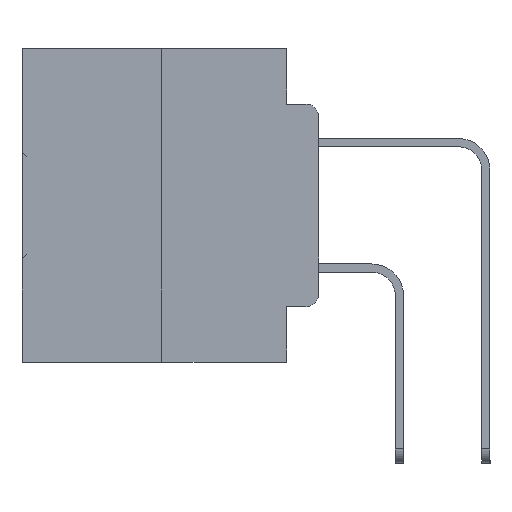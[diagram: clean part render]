
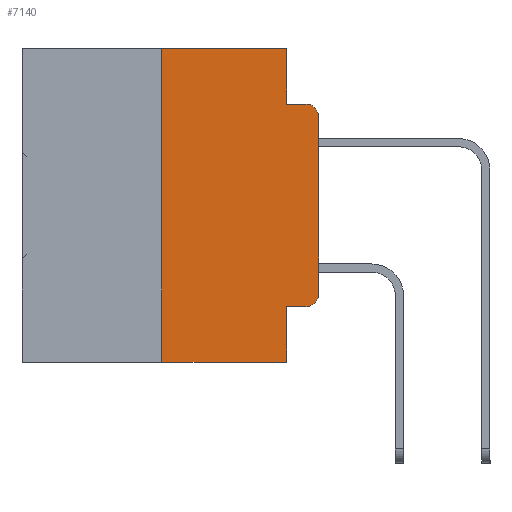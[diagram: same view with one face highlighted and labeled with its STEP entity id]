
A CAD part, left-side view. The second image highlights one B-rep face of the part: STEP entity #7140.
In plain terms, the highlighted planar face has unit normal (-1, 0, 0).
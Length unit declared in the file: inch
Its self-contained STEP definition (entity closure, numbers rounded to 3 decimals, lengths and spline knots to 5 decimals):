
#17 = LINE ( 'NONE', #10587, #12232 ) ;
#778 = VECTOR ( 'NONE', #29544, 39.37008 ) ;
#1004 = VERTEX_POINT ( 'NONE', #22967 ) ;
#1310 = VECTOR ( 'NONE', #13694, 39.37008 ) ;
#1655 = LINE ( 'NONE', #13505, #778 ) ;
#2083 = CIRCLE ( 'NONE', #3443, 0.02 ) ;
#2394 = LINE ( 'NONE', #18961, #31163 ) ;
#2472 = DIRECTION ( 'NONE',  ( 0., -1., 0. ) ) ;
#3310 = CARTESIAN_POINT ( 'NONE',  ( 0., 0.051, 0. ) ) ;
#3443 = AXIS2_PLACEMENT_3D ( 'NONE', #24940, #8804, #27569 ) ;
#3861 = VERTEX_POINT ( 'NONE', #34736 ) ;
#4804 = ORIENTED_EDGE ( 'NONE', *, *, #18585, .T. ) ;
#5105 = DIRECTION ( 'NONE',  ( 0., -1., 0. ) ) ;
#5783 = EDGE_CURVE ( 'NONE', #22459, #1004, #8733, .T. ) ;
#6427 = EDGE_CURVE ( 'NONE', #22459, #11233, #9134, .T. ) ;
#6548 = ORIENTED_EDGE ( 'NONE', *, *, #19818, .F. ) ;
#7105 = LINE ( 'NONE', #26453, #27702 ) ;
#7137 = EDGE_CURVE ( 'NONE', #7697, #31434, #2083, .T. ) ;
#7140 = ADVANCED_FACE ( 'NONE', ( #8635 ), #22324, .F. ) ;
#7409 = CIRCLE ( 'NONE', #26892, 0.02 ) ;
#7697 = VERTEX_POINT ( 'NONE', #21941 ) ;
#7738 = DIRECTION ( 'NONE',  ( 0., 0., -1. ) ) ;
#8262 = VERTEX_POINT ( 'NONE', #34646 ) ;
#8292 = ORIENTED_EDGE ( 'NONE', *, *, #5783, .T. ) ;
#8513 = VERTEX_POINT ( 'NONE', #3310 ) ;
#8619 = DIRECTION ( 'NONE',  ( 0., 0., 1. ) ) ;
#8635 = FACE_OUTER_BOUND ( 'NONE', #21791, .T. ) ;
#8733 = LINE ( 'NONE', #29514, #1310 ) ;
#8804 = DIRECTION ( 'NONE',  ( -1., 0., 0. ) ) ;
#9050 = AXIS2_PLACEMENT_3D ( 'NONE', #14308, #32871, #17050 ) ;
#9134 = LINE ( 'NONE', #19443, #23517 ) ;
#10149 = LINE ( 'NONE', #29936, #30610 ) ;
#10587 = CARTESIAN_POINT ( 'NONE',  ( 0., 0.051, -0.4115 ) ) ;
#11233 = VERTEX_POINT ( 'NONE', #28579 ) ;
#12182 = ORIENTED_EDGE ( 'NONE', *, *, #33385, .T. ) ;
#12232 = VECTOR ( 'NONE', #5105, 39.37008 ) ;
#13505 = CARTESIAN_POINT ( 'NONE',  ( 0., 0., 0. ) ) ;
#13694 = DIRECTION ( 'NONE',  ( 0., -1., 0. ) ) ;
#14308 = CARTESIAN_POINT ( 'NONE',  ( 0., 0.473, 0. ) ) ;
#16082 = CARTESIAN_POINT ( 'NONE',  ( 0., 0.25, -0.5 ) ) ;
#16399 = DIRECTION ( 'NONE',  ( -1., 0., 0. ) ) ;
#17050 = DIRECTION ( 'NONE',  ( 0., 0., -1. ) ) ;
#18585 = EDGE_CURVE ( 'NONE', #31434, #26821, #1655, .T. ) ;
#18961 = CARTESIAN_POINT ( 'NONE',  ( 0., 0.473, 0. ) ) ;
#19443 = CARTESIAN_POINT ( 'NONE',  ( 0., 0.25, 0. ) ) ;
#19786 = ORIENTED_EDGE ( 'NONE', *, *, #7137, .T. ) ;
#19818 = EDGE_CURVE ( 'NONE', #11233, #8513, #2394, .T. ) ;
#21057 = ORIENTED_EDGE ( 'NONE', *, *, #6427, .F. ) ;
#21791 = EDGE_LOOP ( 'NONE', ( #4804, #12182, #26392, #27194, #6548, #21057, #8292, #24343, #25158, #19786 ) ) ;
#21941 = CARTESIAN_POINT ( 'NONE',  ( 0., 0.02, -0.4115 ) ) ;
#22324 = PLANE ( 'NONE',  #9050 ) ;
#22459 = VERTEX_POINT ( 'NONE', #16082 ) ;
#22967 = CARTESIAN_POINT ( 'NONE',  ( 0., 0.051, -0.5 ) ) ;
#23188 = LINE ( 'NONE', #24961, #30134 ) ;
#23517 = VECTOR ( 'NONE', #8619, 39.37008 ) ;
#24343 = ORIENTED_EDGE ( 'NONE', *, *, #32271, .F. ) ;
#24565 = EDGE_CURVE ( 'NONE', #8513, #3861, #7105, .T. ) ;
#24940 = CARTESIAN_POINT ( 'NONE',  ( 0., 0.02, -0.3915 ) ) ;
#24961 = CARTESIAN_POINT ( 'NONE',  ( 0., 0.051, 0. ) ) ;
#25158 = ORIENTED_EDGE ( 'NONE', *, *, #25221, .T. ) ;
#25221 = EDGE_CURVE ( 'NONE', #8262, #7697, #17, .T. ) ;
#26392 = ORIENTED_EDGE ( 'NONE', *, *, #31637, .F. ) ;
#26453 = CARTESIAN_POINT ( 'NONE',  ( 0., 0.051, 0. ) ) ;
#26821 = VERTEX_POINT ( 'NONE', #29969 ) ;
#26892 = AXIS2_PLACEMENT_3D ( 'NONE', #32252, #16399, #34901 ) ;
#27194 = ORIENTED_EDGE ( 'NONE', *, *, #24565, .F. ) ;
#27394 = DIRECTION ( 'NONE',  ( 0., -1., 0. ) ) ;
#27486 = DIRECTION ( 'NONE',  ( 0., 0., -1. ) ) ;
#27500 = VERTEX_POINT ( 'NONE', #32920 ) ;
#27569 = DIRECTION ( 'NONE',  ( 0., 0., -1. ) ) ;
#27702 = VECTOR ( 'NONE', #7738, 39.37008 ) ;
#28579 = CARTESIAN_POINT ( 'NONE',  ( 0., 0.25, 0. ) ) ;
#29514 = CARTESIAN_POINT ( 'NONE',  ( 0., 0.473, -0.5 ) ) ;
#29544 = DIRECTION ( 'NONE',  ( 0., 0., 1. ) ) ;
#29936 = CARTESIAN_POINT ( 'NONE',  ( 0., 0.051, -0.0885 ) ) ;
#29969 = CARTESIAN_POINT ( 'NONE',  ( 0., 0., -0.1085 ) ) ;
#30134 = VECTOR ( 'NONE', #27486, 39.37008 ) ;
#30610 = VECTOR ( 'NONE', #27394, 39.37008 ) ;
#31163 = VECTOR ( 'NONE', #2472, 39.37008 ) ;
#31216 = CARTESIAN_POINT ( 'NONE',  ( 0., 0., -0.3915 ) ) ;
#31434 = VERTEX_POINT ( 'NONE', #31216 ) ;
#31637 = EDGE_CURVE ( 'NONE', #3861, #27500, #10149, .T. ) ;
#32252 = CARTESIAN_POINT ( 'NONE',  ( 0., 0.02, -0.1085 ) ) ;
#32271 = EDGE_CURVE ( 'NONE', #8262, #1004, #23188, .T. ) ;
#32871 = DIRECTION ( 'NONE',  ( 1., 0., 0. ) ) ;
#32920 = CARTESIAN_POINT ( 'NONE',  ( 0., 0.02, -0.0885 ) ) ;
#33385 = EDGE_CURVE ( 'NONE', #26821, #27500, #7409, .T. ) ;
#34646 = CARTESIAN_POINT ( 'NONE',  ( 0., 0.051, -0.4115 ) ) ;
#34736 = CARTESIAN_POINT ( 'NONE',  ( 0., 0.051, -0.0885 ) ) ;
#34901 = DIRECTION ( 'NONE',  ( 0., 0., -1. ) ) ;
